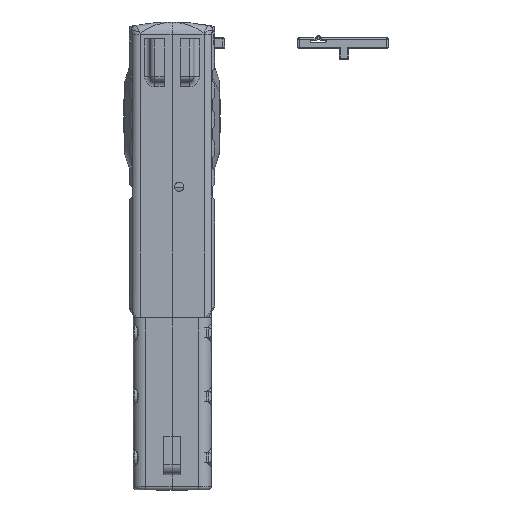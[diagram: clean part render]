
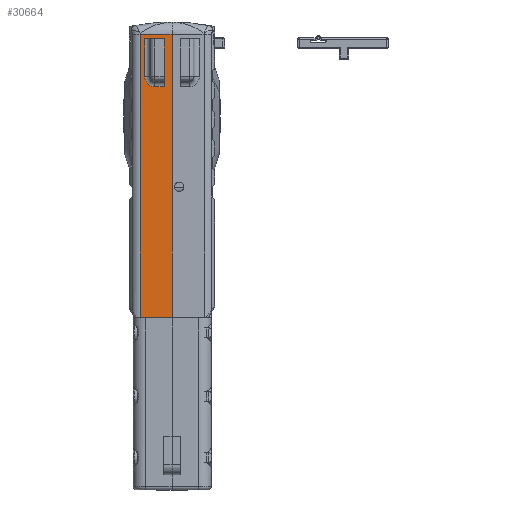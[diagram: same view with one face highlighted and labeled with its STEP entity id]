
A CAD part, top view. The second image highlights one B-rep face of the part: STEP entity #30664.
In plain terms, the highlighted planar face has unit normal (0, 0, 1).
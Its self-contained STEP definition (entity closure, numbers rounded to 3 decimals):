
#613=FACE_BOUND($,#10405,.T.);
#1172=PLANE($,#32901);
#2875=LINE($,#44865,#5422);
#2936=LINE($,#45430,#5483);
#2942=LINE($,#45466,#5489);
#2943=LINE($,#45505,#5490);
#2953=LINE($,#45650,#5500);
#2954=LINE($,#45652,#5501);
#2955=LINE($,#45656,#5502);
#2956=LINE($,#45657,#5503);
#5422=VECTOR($,#36259,12.073);
#5483=VECTOR($,#36476,12.073);
#5489=VECTOR($,#36484,1.366);
#5490=VECTOR($,#36489,1.366);
#5500=VECTOR($,#36549,2.041);
#5501=VECTOR($,#36550,0.39);
#5502=VECTOR($,#36553,1.609);
#5503=VECTOR($,#36554,0.822);
#8552=FACE_OUTER_BOUND($,#10404,.T.);
#10404=EDGE_LOOP($,(#22168,#22169,#22170,#22171));
#10405=EDGE_LOOP($,(#22172,#22173,#22174,#22175,#22176));
#12703=CIRCLE($,#32902,0.432);
#13859=VERTEX_POINT($,#44862);
#13860=VERTEX_POINT($,#44864);
#13943=VERTEX_POINT($,#45421);
#13944=VERTEX_POINT($,#45428);
#13964=VERTEX_POINT($,#45648);
#13965=VERTEX_POINT($,#45649);
#13966=VERTEX_POINT($,#45651);
#13967=VERTEX_POINT($,#45653);
#13968=VERTEX_POINT($,#45655);
#16960=EDGE_CURVE($,#13859,#13860,#2875,.T.);
#17087=EDGE_CURVE($,#13944,#13943,#2936,.T.);
#17095=EDGE_CURVE($,#13860,#13944,#2942,.T.);
#17098=EDGE_CURVE($,#13943,#13859,#2943,.T.);
#17124=EDGE_CURVE($,#13964,#13965,#2953,.T.);
#17125=EDGE_CURVE($,#13965,#13966,#2954,.T.);
#17126=EDGE_CURVE($,#13967,#13966,#12703,.T.);
#17127=EDGE_CURVE($,#13967,#13968,#2955,.T.);
#17128=EDGE_CURVE($,#13968,#13964,#2956,.T.);
#22168=ORIENTED_EDGE($,*,*,#17087,.F.);
#22169=ORIENTED_EDGE($,*,*,#17095,.F.);
#22170=ORIENTED_EDGE($,*,*,#16960,.F.);
#22171=ORIENTED_EDGE($,*,*,#17098,.F.);
#22172=ORIENTED_EDGE($,*,*,#17124,.T.);
#22173=ORIENTED_EDGE($,*,*,#17125,.T.);
#22174=ORIENTED_EDGE($,*,*,#17126,.F.);
#22175=ORIENTED_EDGE($,*,*,#17127,.T.);
#22176=ORIENTED_EDGE($,*,*,#17128,.T.);
#30664=ADVANCED_FACE($,(#8552,#613),#1172,.T.);
#32901=AXIS2_PLACEMENT_3D($,#45647,#36547,#36548);
#32902=AXIS2_PLACEMENT_3D($,#45654,#36551,#36552);
#36259=DIRECTION($,(0.,-1.,0.));
#36476=DIRECTION($,(0.,1.,0.));
#36484=DIRECTION($,(-1.,0.,0.));
#36489=DIRECTION($,(1.,0.,0.));
#36547=DIRECTION('center_axis',(0.,0.,1.));
#36548=DIRECTION('ref_axis',(0.,1.,0.));
#36549=DIRECTION($,(0.,-1.,0.));
#36550=DIRECTION($,(-1.,0.,0.));
#36551=DIRECTION('center_axis',(0.,0.,1.));
#36552=DIRECTION('ref_axis',(1.,0.,0.));
#36553=DIRECTION($,(0.,1.,0.));
#36554=DIRECTION($,(1.,0.,0.));
#44862=CARTESIAN_POINT('',(-18.551,20.921,14.052));
#44864=CARTESIAN_POINT('',(-18.551,8.847,14.052));
#44865=CARTESIAN_POINT($,(-18.551,11.713,14.052));
#45421=CARTESIAN_POINT('',(-19.917,20.921,14.052));
#45428=CARTESIAN_POINT('',(-19.917,8.847,14.052));
#45430=CARTESIAN_POINT($,(-19.917,1.471,14.052));
#45466=CARTESIAN_POINT($,(-15.402,8.847,14.052));
#45505=CARTESIAN_POINT($,(-12.253,20.921,14.052));
#45647=CARTESIAN_POINT('Origin',(-12.253,10.047,14.052));
#45648=CARTESIAN_POINT('',(-18.892,20.733,14.052));
#45649=CARTESIAN_POINT('',(-18.892,18.692,14.052));
#45650=CARTESIAN_POINT($,(-18.892,15.086,14.052));
#45651=CARTESIAN_POINT('',(-19.282,18.692,14.052));
#45652=CARTESIAN_POINT($,(-19.217,18.692,14.052));
#45653=CARTESIAN_POINT('',(-19.714,19.124,14.052));
#45654=CARTESIAN_POINT('Origin',(-19.282,19.124,14.052));
#45655=CARTESIAN_POINT('',(-19.714,20.733,14.052));
#45656=CARTESIAN_POINT($,(-19.714,20.89,14.052));
#45657=CARTESIAN_POINT($,(-16.74,20.733,14.052));
